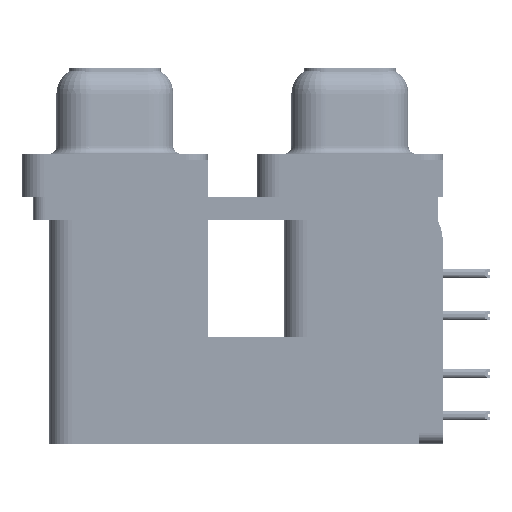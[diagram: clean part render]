
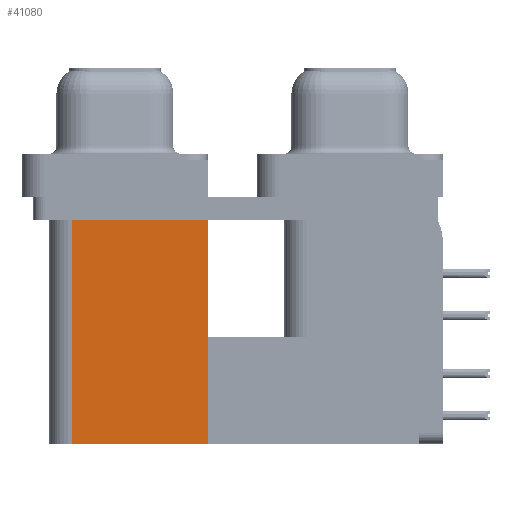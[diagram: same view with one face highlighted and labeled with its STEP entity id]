
A CAD part, left-side view. The second image highlights one B-rep face of the part: STEP entity #41080.
In plain terms, the highlighted planar face has unit normal (-1, 0, 0).
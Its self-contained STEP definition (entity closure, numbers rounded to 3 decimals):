
#822 = EDGE_CURVE ( 'NONE', #16070, #33611, #31719, .T. ) ;
#1276 = ORIENTED_EDGE ( 'NONE', *, *, #48948, .T. ) ;
#2275 = DIRECTION ( 'NONE',  ( 0., 1., 0. ) ) ;
#4325 = LINE ( 'NONE', #40160, #49618 ) ;
#4641 = CARTESIAN_POINT ( 'NONE',  ( 3.7, 9.6, -2.5 ) ) ;
#10802 = LINE ( 'NONE', #42509, #31446 ) ;
#11013 = EDGE_LOOP ( 'NONE', ( #1276, #24663, #52480, #14342 ) ) ;
#13502 = CARTESIAN_POINT ( 'NONE',  ( 3.7, 9.6, -19.2 ) ) ;
#14342 = ORIENTED_EDGE ( 'NONE', *, *, #57596, .T. ) ;
#16070 = VERTEX_POINT ( 'NONE', #24642 ) ;
#16296 = FACE_OUTER_BOUND ( 'NONE', #11013, .T. ) ;
#18553 = CARTESIAN_POINT ( 'NONE',  ( 3.7, 18.8, -2.5 ) ) ;
#21737 = DIRECTION ( 'NONE',  ( 0., 1., 0. ) ) ;
#24642 = CARTESIAN_POINT ( 'NONE',  ( 3.7, 9.6, -19.2 ) ) ;
#24663 = ORIENTED_EDGE ( 'NONE', *, *, #37838, .F. ) ;
#24886 = VECTOR ( 'NONE', #35186, 1000. ) ;
#25127 = CARTESIAN_POINT ( 'NONE',  ( 3.7, 9.6, -19.2 ) ) ;
#27218 = VERTEX_POINT ( 'NONE', #4641 ) ;
#28969 = AXIS2_PLACEMENT_3D ( 'NONE', #25127, #55950, #51285 ) ;
#30193 = CARTESIAN_POINT ( 'NONE',  ( 3.7, 18.8, -19.2 ) ) ;
#31446 = VECTOR ( 'NONE', #2275, 1000. ) ;
#31719 = LINE ( 'NONE', #13502, #54387 ) ;
#33611 = VERTEX_POINT ( 'NONE', #54609 ) ;
#35186 = DIRECTION ( 'NONE',  ( 0., 0., 1. ) ) ;
#35784 = DIRECTION ( 'NONE',  ( 0., 0., 1. ) ) ;
#37785 = PLANE ( 'NONE',  #28969 ) ;
#37838 = EDGE_CURVE ( 'NONE', #33611, #56934, #40147, .T. ) ;
#40147 = LINE ( 'NONE', #30193, #24886 ) ;
#40160 = CARTESIAN_POINT ( 'NONE',  ( 3.7, 9.6, -19.2 ) ) ;
#41080 = ADVANCED_FACE ( 'NONE', ( #16296 ), #37785, .F. ) ;
#42509 = CARTESIAN_POINT ( 'NONE',  ( 3.7, 9.6, -2.5 ) ) ;
#48948 = EDGE_CURVE ( 'NONE', #27218, #56934, #10802, .T. ) ;
#49618 = VECTOR ( 'NONE', #35784, 1000. ) ;
#51285 = DIRECTION ( 'NONE',  ( 0., 1., 0. ) ) ;
#52480 = ORIENTED_EDGE ( 'NONE', *, *, #822, .F. ) ;
#54387 = VECTOR ( 'NONE', #21737, 1000. ) ;
#54609 = CARTESIAN_POINT ( 'NONE',  ( 3.7, 18.8, -19.2 ) ) ;
#55950 = DIRECTION ( 'NONE',  ( 1., 0., 0. ) ) ;
#56934 = VERTEX_POINT ( 'NONE', #18553 ) ;
#57596 = EDGE_CURVE ( 'NONE', #16070, #27218, #4325, .T. ) ;
